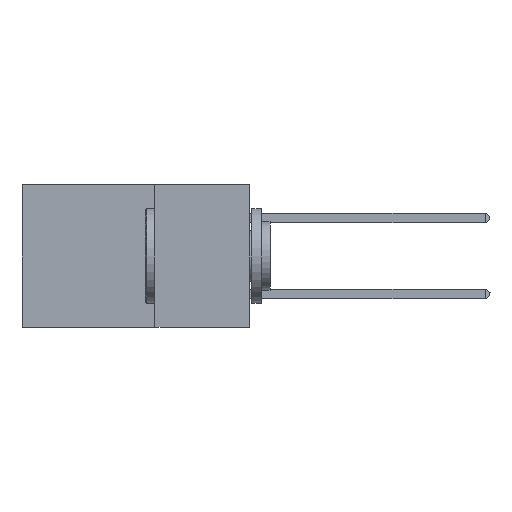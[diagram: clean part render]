
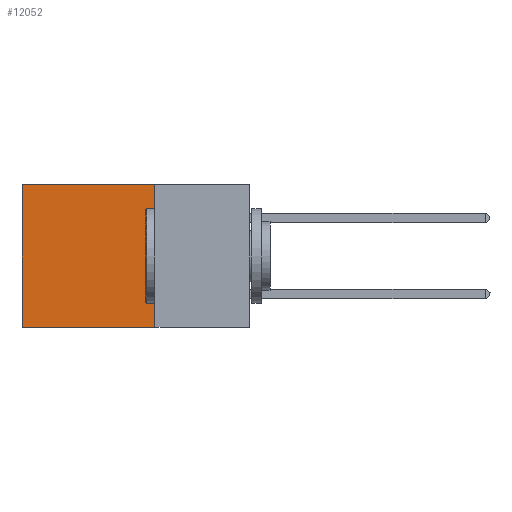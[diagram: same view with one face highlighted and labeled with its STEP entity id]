
A CAD part, left-side view. The second image highlights one B-rep face of the part: STEP entity #12052.
In plain terms, the highlighted planar face has unit normal (-1, 0, 0).
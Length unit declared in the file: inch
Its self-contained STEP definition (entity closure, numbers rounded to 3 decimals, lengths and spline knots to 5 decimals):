
#69 = DIRECTION ( 'NONE',  ( 0., 1., 0. ) ) ;
#960 = VECTOR ( 'NONE', #69, 39.37008 ) ;
#2627 = EDGE_CURVE ( 'NONE', #2760, #13365, #14457, .T. ) ;
#2760 = VERTEX_POINT ( 'NONE', #21383 ) ;
#3790 = LINE ( 'NONE', #16242, #9819 ) ;
#3914 = EDGE_CURVE ( 'NONE', #2760, #14775, #10524, .T. ) ;
#4096 = DIRECTION ( 'NONE',  ( 0., 0., -1. ) ) ;
#4214 = FACE_OUTER_BOUND ( 'NONE', #4311, .T. ) ;
#4311 = EDGE_LOOP ( 'NONE', ( #15689, #4320, #15923, #4970 ) ) ;
#4320 = ORIENTED_EDGE ( 'NONE', *, *, #4716, .F. ) ;
#4716 = EDGE_CURVE ( 'NONE', #13365, #18523, #20309, .T. ) ;
#4970 = ORIENTED_EDGE ( 'NONE', *, *, #3914, .T. ) ;
#5216 = CARTESIAN_POINT ( 'NONE',  ( 0.2875, 0.6, -0.375 ) ) ;
#6213 = VECTOR ( 'NONE', #17758, 39.37008 ) ;
#6457 = CARTESIAN_POINT ( 'NONE',  ( 0.2875, 0.25, -0.375 ) ) ;
#7033 = AXIS2_PLACEMENT_3D ( 'NONE', #6457, #15352, #20577 ) ;
#8452 = EDGE_CURVE ( 'NONE', #14775, #18523, #3790, .T. ) ;
#8769 = CARTESIAN_POINT ( 'NONE',  ( 0.2875, 0.25, 0. ) ) ;
#8976 = CARTESIAN_POINT ( 'NONE',  ( 0.2875, 0.25, -0.375 ) ) ;
#9819 = VECTOR ( 'NONE', #4096, 39.37008 ) ;
#10524 = LINE ( 'NONE', #8769, #960 ) ;
#12052 = ADVANCED_FACE ( 'NONE', ( #4214 ), #13585, .F. ) ;
#12962 = VECTOR ( 'NONE', #17767, 39.37008 ) ;
#13365 = VERTEX_POINT ( 'NONE', #22041 ) ;
#13585 = PLANE ( 'NONE',  #7033 ) ;
#14457 = LINE ( 'NONE', #8976, #6213 ) ;
#14775 = VERTEX_POINT ( 'NONE', #17613 ) ;
#15352 = DIRECTION ( 'NONE',  ( 1., 0., 0. ) ) ;
#15689 = ORIENTED_EDGE ( 'NONE', *, *, #8452, .T. ) ;
#15923 = ORIENTED_EDGE ( 'NONE', *, *, #2627, .F. ) ;
#16242 = CARTESIAN_POINT ( 'NONE',  ( 0.2875, 0.6, -0.375 ) ) ;
#16598 = CARTESIAN_POINT ( 'NONE',  ( 0.2875, 0.25, -0.375 ) ) ;
#17613 = CARTESIAN_POINT ( 'NONE',  ( 0.2875, 0.6, 0. ) ) ;
#17758 = DIRECTION ( 'NONE',  ( 0., 0., -1. ) ) ;
#17767 = DIRECTION ( 'NONE',  ( 0., 1., 0. ) ) ;
#18523 = VERTEX_POINT ( 'NONE', #5216 ) ;
#20309 = LINE ( 'NONE', #16598, #12962 ) ;
#20577 = DIRECTION ( 'NONE',  ( 0., 0., -1. ) ) ;
#21383 = CARTESIAN_POINT ( 'NONE',  ( 0.2875, 0.25, 0. ) ) ;
#22041 = CARTESIAN_POINT ( 'NONE',  ( 0.2875, 0.25, -0.375 ) ) ;
